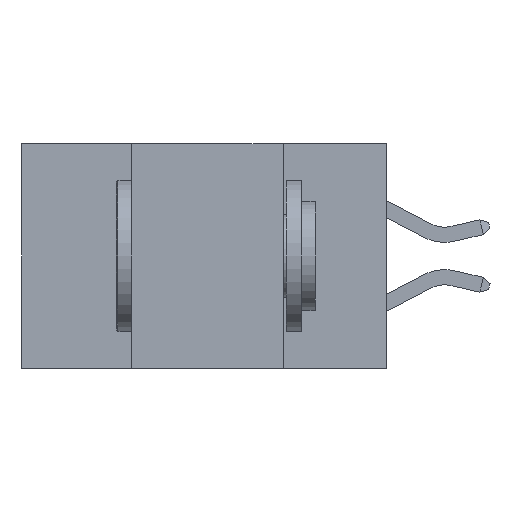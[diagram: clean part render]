
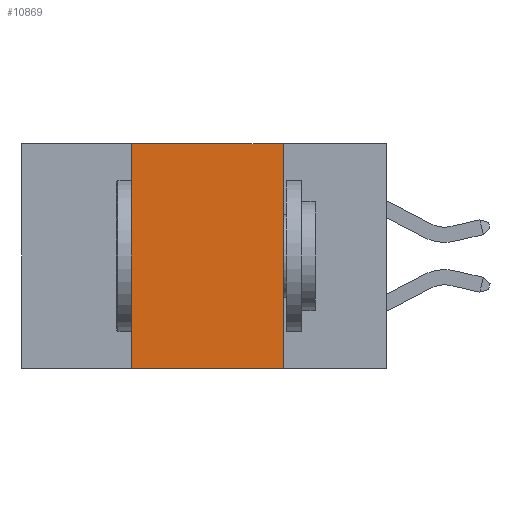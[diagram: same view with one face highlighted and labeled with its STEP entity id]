
A CAD part, left-side view. The second image highlights one B-rep face of the part: STEP entity #10869.
In plain terms, the highlighted planar face has unit normal (-1, 0, 0).
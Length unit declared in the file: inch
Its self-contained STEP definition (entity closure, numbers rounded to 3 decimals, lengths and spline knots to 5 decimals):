
#481 = VECTOR ( 'NONE', #10566, 39.37008 ) ;
#1180 = FACE_OUTER_BOUND ( 'NONE', #3154, .T. ) ;
#1423 = CARTESIAN_POINT ( 'NONE',  ( 0., 0.17, 0. ) ) ;
#1458 = CARTESIAN_POINT ( 'NONE',  ( 0., 0.42, 0. ) ) ;
#1948 = DIRECTION ( 'NONE',  ( 0., -1., 0. ) ) ;
#2369 = LINE ( 'NONE', #2426, #9725 ) ;
#2426 = CARTESIAN_POINT ( 'NONE',  ( 0., 0.6, -0.37 ) ) ;
#2456 = VERTEX_POINT ( 'NONE', #1423 ) ;
#2527 = EDGE_CURVE ( 'NONE', #2910, #10056, #2369, .T. ) ;
#2537 = CARTESIAN_POINT ( 'NONE',  ( 0., 0.17, 0. ) ) ;
#2910 = VERTEX_POINT ( 'NONE', #12063 ) ;
#3154 = EDGE_LOOP ( 'NONE', ( #11942, #10152, #9839, #11547 ) ) ;
#3310 = DIRECTION ( 'NONE',  ( 1., 0., 0. ) ) ;
#3538 = VECTOR ( 'NONE', #1948, 39.37008 ) ;
#3587 = LINE ( 'NONE', #1458, #481 ) ;
#4288 = PLANE ( 'NONE',  #4778 ) ;
#4334 = CARTESIAN_POINT ( 'NONE',  ( 0., 0.6, 0. ) ) ;
#4463 = VECTOR ( 'NONE', #5471, 39.37008 ) ;
#4643 = CARTESIAN_POINT ( 'NONE',  ( 0., 0.42, 0. ) ) ;
#4778 = AXIS2_PLACEMENT_3D ( 'NONE', #4334, #3310, #10374 ) ;
#5471 = DIRECTION ( 'NONE',  ( 0., 0., -1. ) ) ;
#5485 = DIRECTION ( 'NONE',  ( 0., -1., 0. ) ) ;
#5655 = EDGE_CURVE ( 'NONE', #2910, #9117, #3587, .T. ) ;
#6193 = LINE ( 'NONE', #9831, #3538 ) ;
#7521 = EDGE_CURVE ( 'NONE', #9117, #2456, #6193, .T. ) ;
#9010 = EDGE_CURVE ( 'NONE', #2456, #10056, #9787, .T. ) ;
#9117 = VERTEX_POINT ( 'NONE', #4643 ) ;
#9725 = VECTOR ( 'NONE', #5485, 39.37008 ) ;
#9787 = LINE ( 'NONE', #2537, #4463 ) ;
#9831 = CARTESIAN_POINT ( 'NONE',  ( 0., 0.6, 0. ) ) ;
#9839 = ORIENTED_EDGE ( 'NONE', *, *, #5655, .F. ) ;
#10056 = VERTEX_POINT ( 'NONE', #11016 ) ;
#10152 = ORIENTED_EDGE ( 'NONE', *, *, #7521, .F. ) ;
#10374 = DIRECTION ( 'NONE',  ( 0., 0., -1. ) ) ;
#10566 = DIRECTION ( 'NONE',  ( 0., 0., 1. ) ) ;
#10869 = ADVANCED_FACE ( 'NONE', ( #1180 ), #4288, .F. ) ;
#11016 = CARTESIAN_POINT ( 'NONE',  ( 0., 0.17, -0.37 ) ) ;
#11547 = ORIENTED_EDGE ( 'NONE', *, *, #2527, .T. ) ;
#11942 = ORIENTED_EDGE ( 'NONE', *, *, #9010, .F. ) ;
#12063 = CARTESIAN_POINT ( 'NONE',  ( 0., 0.42, -0.37 ) ) ;
